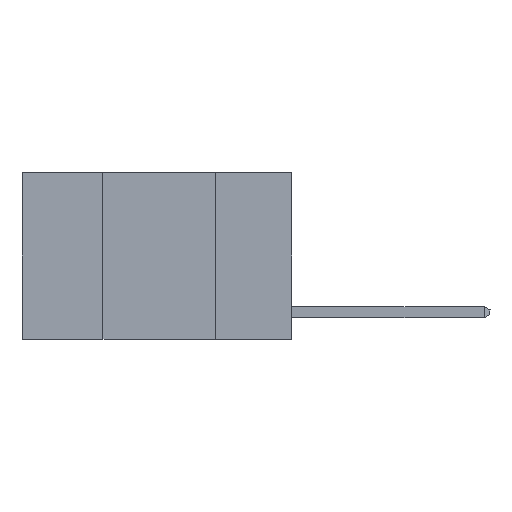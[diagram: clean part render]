
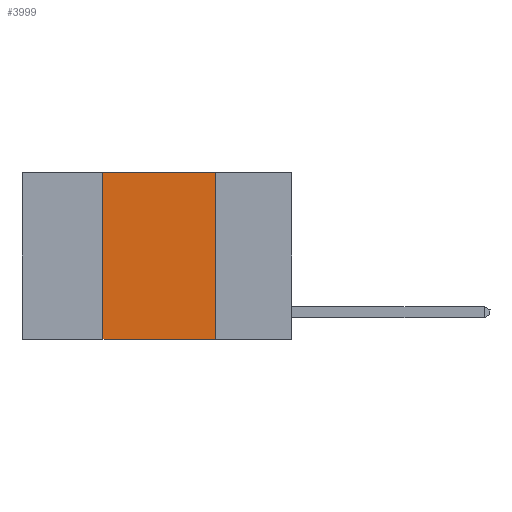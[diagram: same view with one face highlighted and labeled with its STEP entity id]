
A CAD part, left-side view. The second image highlights one B-rep face of the part: STEP entity #3999.
In plain terms, the highlighted planar face has unit normal (-1, 0, 0).
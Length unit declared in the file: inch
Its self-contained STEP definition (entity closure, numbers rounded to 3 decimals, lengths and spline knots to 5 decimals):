
#873 = DIRECTION ( 'NONE',  ( 0., 0., -1. ) ) ;
#929 = ORIENTED_EDGE ( 'NONE', *, *, #3541, .F. ) ;
#985 = CARTESIAN_POINT ( 'NONE',  ( 0., 0.42, -0.37 ) ) ;
#1660 = VERTEX_POINT ( 'NONE', #14466 ) ;
#1905 = EDGE_CURVE ( 'NONE', #15509, #1660, #3900, .T. ) ;
#2657 = VERTEX_POINT ( 'NONE', #13823 ) ;
#3008 = EDGE_CURVE ( 'NONE', #15509, #2657, #13905, .T. ) ;
#3426 = VECTOR ( 'NONE', #5394, 39.37008 ) ;
#3497 = CARTESIAN_POINT ( 'NONE',  ( 0., 0.17, 0. ) ) ;
#3541 = EDGE_CURVE ( 'NONE', #6757, #1660, #3552, .T. ) ;
#3552 = LINE ( 'NONE', #7589, #11817 ) ;
#3900 = LINE ( 'NONE', #8888, #8286 ) ;
#3999 = ADVANCED_FACE ( 'NONE', ( #20380 ), #16871, .F. ) ;
#4094 = VECTOR ( 'NONE', #9556, 39.37008 ) ;
#4418 = ORIENTED_EDGE ( 'NONE', *, *, #3008, .F. ) ;
#4823 = ORIENTED_EDGE ( 'NONE', *, *, #1905, .T. ) ;
#5394 = DIRECTION ( 'NONE',  ( 0., -1., 0. ) ) ;
#5429 = CARTESIAN_POINT ( 'NONE',  ( 0., 0.6, 0. ) ) ;
#6333 = CARTESIAN_POINT ( 'NONE',  ( 0., 0.42, 0. ) ) ;
#6757 = VERTEX_POINT ( 'NONE', #3497 ) ;
#7589 = CARTESIAN_POINT ( 'NONE',  ( 0., 0.17, 0. ) ) ;
#8286 = VECTOR ( 'NONE', #8794, 39.37008 ) ;
#8732 = DIRECTION ( 'NONE',  ( 0., 0., -1. ) ) ;
#8794 = DIRECTION ( 'NONE',  ( 0., -1., 0. ) ) ;
#8888 = CARTESIAN_POINT ( 'NONE',  ( 0., 0.6, -0.37 ) ) ;
#9556 = DIRECTION ( 'NONE',  ( 0., 0., 1. ) ) ;
#10170 = ORIENTED_EDGE ( 'NONE', *, *, #15919, .F. ) ;
#11817 = VECTOR ( 'NONE', #873, 39.37008 ) ;
#13823 = CARTESIAN_POINT ( 'NONE',  ( 0., 0.42, 0. ) ) ;
#13905 = LINE ( 'NONE', #6333, #4094 ) ;
#14466 = CARTESIAN_POINT ( 'NONE',  ( 0., 0.17, -0.37 ) ) ;
#15210 = CARTESIAN_POINT ( 'NONE',  ( 0., 0.6, 0. ) ) ;
#15509 = VERTEX_POINT ( 'NONE', #985 ) ;
#15919 = EDGE_CURVE ( 'NONE', #2657, #6757, #20766, .T. ) ;
#16871 = PLANE ( 'NONE',  #20910 ) ;
#18482 = DIRECTION ( 'NONE',  ( 1., 0., 0. ) ) ;
#18581 = EDGE_LOOP ( 'NONE', ( #929, #10170, #4418, #4823 ) ) ;
#20380 = FACE_OUTER_BOUND ( 'NONE', #18581, .T. ) ;
#20766 = LINE ( 'NONE', #15210, #3426 ) ;
#20910 = AXIS2_PLACEMENT_3D ( 'NONE', #5429, #18482, #8732 ) ;
